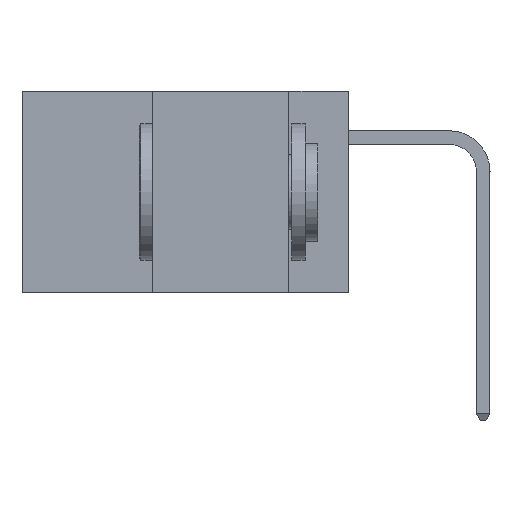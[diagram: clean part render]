
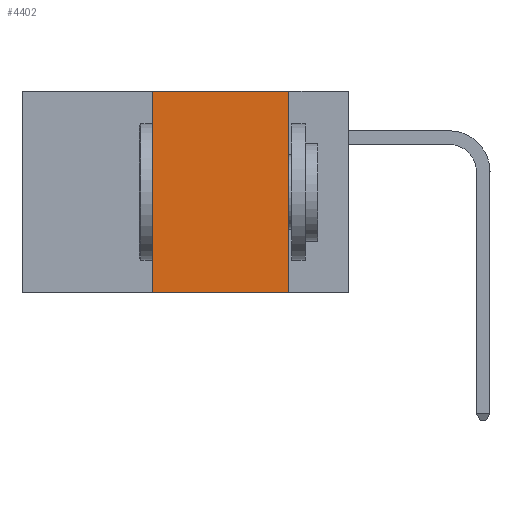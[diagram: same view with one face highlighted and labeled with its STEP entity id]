
A CAD part, left-side view. The second image highlights one B-rep face of the part: STEP entity #4402.
In plain terms, the highlighted planar face has unit normal (-1, 0, 0).
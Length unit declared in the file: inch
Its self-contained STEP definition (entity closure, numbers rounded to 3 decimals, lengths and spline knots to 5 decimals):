
#559 = EDGE_LOOP ( 'NONE', ( #43907, #21114, #31930, #6427 ) ) ;
#2272 = LINE ( 'NONE', #8371, #25343 ) ;
#3646 = EDGE_CURVE ( 'NONE', #17673, #16651, #45149, .T. ) ;
#4402 = ADVANCED_FACE ( 'NONE', ( #21423 ), #5019, .F. ) ;
#5019 = PLANE ( 'NONE',  #14351 ) ;
#6427 = ORIENTED_EDGE ( 'NONE', *, *, #35058, .T. ) ;
#8371 = CARTESIAN_POINT ( 'NONE',  ( 0., 0.11, 0. ) ) ;
#8400 = CARTESIAN_POINT ( 'NONE',  ( 0., 0.6, 0. ) ) ;
#10455 = CARTESIAN_POINT ( 'NONE',  ( 0., 0.6, 0. ) ) ;
#12555 = CARTESIAN_POINT ( 'NONE',  ( 0., 0.36, -0.37 ) ) ;
#14275 = CARTESIAN_POINT ( 'NONE',  ( 0., 0.36, 0. ) ) ;
#14351 = AXIS2_PLACEMENT_3D ( 'NONE', #8400, #36463, #31871 ) ;
#15551 = CARTESIAN_POINT ( 'NONE',  ( 0., 0.11, 0. ) ) ;
#16651 = VERTEX_POINT ( 'NONE', #15551 ) ;
#17673 = VERTEX_POINT ( 'NONE', #36214 ) ;
#18796 = VERTEX_POINT ( 'NONE', #36549 ) ;
#21114 = ORIENTED_EDGE ( 'NONE', *, *, #3646, .F. ) ;
#21423 = FACE_OUTER_BOUND ( 'NONE', #559, .T. ) ;
#21634 = LINE ( 'NONE', #14275, #22765 ) ;
#22471 = VECTOR ( 'NONE', #44651, 39.37008 ) ;
#22721 = VERTEX_POINT ( 'NONE', #12555 ) ;
#22765 = VECTOR ( 'NONE', #28368, 39.37008 ) ;
#25018 = DIRECTION ( 'NONE',  ( 0., -1., 0. ) ) ;
#25343 = VECTOR ( 'NONE', #25598, 39.37008 ) ;
#25598 = DIRECTION ( 'NONE',  ( 0., 0., -1. ) ) ;
#28368 = DIRECTION ( 'NONE',  ( 0., 0., 1. ) ) ;
#29852 = EDGE_CURVE ( 'NONE', #16651, #18796, #2272, .T. ) ;
#31871 = DIRECTION ( 'NONE',  ( 0., 0., -1. ) ) ;
#31930 = ORIENTED_EDGE ( 'NONE', *, *, #37948, .F. ) ;
#35058 = EDGE_CURVE ( 'NONE', #22721, #18796, #39989, .T. ) ;
#35774 = VECTOR ( 'NONE', #25018, 39.37008 ) ;
#36214 = CARTESIAN_POINT ( 'NONE',  ( 0., 0.36, 0. ) ) ;
#36463 = DIRECTION ( 'NONE',  ( 1., 0., 0. ) ) ;
#36549 = CARTESIAN_POINT ( 'NONE',  ( 0., 0.11, -0.37 ) ) ;
#36964 = CARTESIAN_POINT ( 'NONE',  ( 0., 0.6, -0.37 ) ) ;
#37948 = EDGE_CURVE ( 'NONE', #22721, #17673, #21634, .T. ) ;
#39989 = LINE ( 'NONE', #36964, #22471 ) ;
#43907 = ORIENTED_EDGE ( 'NONE', *, *, #29852, .F. ) ;
#44651 = DIRECTION ( 'NONE',  ( 0., -1., 0. ) ) ;
#45149 = LINE ( 'NONE', #10455, #35774 ) ;
